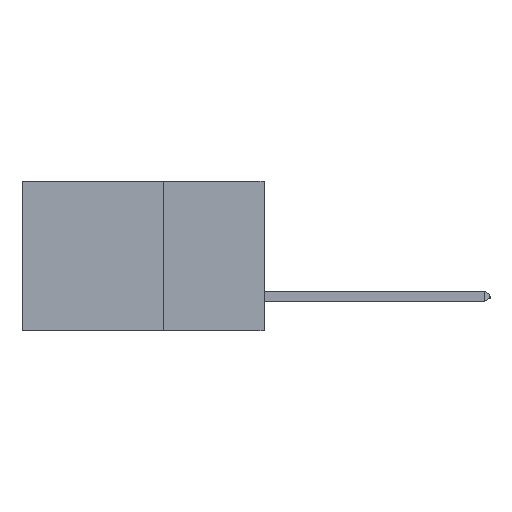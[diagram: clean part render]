
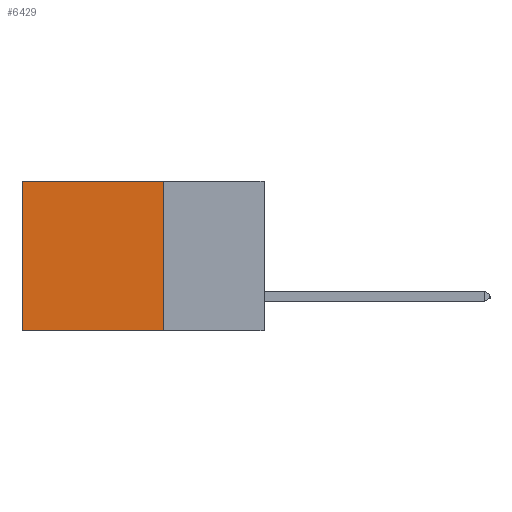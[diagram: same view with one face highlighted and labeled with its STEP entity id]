
A CAD part, left-side view. The second image highlights one B-rep face of the part: STEP entity #6429.
In plain terms, the highlighted planar face has unit normal (-1, 0, 0).
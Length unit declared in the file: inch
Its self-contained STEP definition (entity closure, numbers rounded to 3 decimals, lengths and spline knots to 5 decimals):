
#292 = AXIS2_PLACEMENT_3D ( 'NONE', #7613, #2351, #9661 ) ;
#304 = VECTOR ( 'NONE', #11605, 39.37008 ) ;
#675 = ORIENTED_EDGE ( 'NONE', *, *, #13280, .T. ) ;
#685 = DIRECTION ( 'NONE',  ( 0., 0., -1. ) ) ;
#794 = EDGE_CURVE ( 'NONE', #12680, #6023, #10056, .T. ) ;
#941 = CARTESIAN_POINT ( 'NONE',  ( 0.298, 0.25, 0. ) ) ;
#1238 = PLANE ( 'NONE',  #292 ) ;
#1508 = CARTESIAN_POINT ( 'NONE',  ( 0.298, 0.6, -0.37 ) ) ;
#2351 = DIRECTION ( 'NONE',  ( 1., 0., 0. ) ) ;
#2764 = CARTESIAN_POINT ( 'NONE',  ( 0.298, 0.25, -0.37 ) ) ;
#3000 = EDGE_LOOP ( 'NONE', ( #675, #11033, #6759, #5503 ) ) ;
#3111 = VERTEX_POINT ( 'NONE', #1508 ) ;
#3615 = CARTESIAN_POINT ( 'NONE',  ( 0.298, 0.25, 0. ) ) ;
#3887 = VECTOR ( 'NONE', #685, 39.37008 ) ;
#4018 = CARTESIAN_POINT ( 'NONE',  ( 0.298, 0.6, 0. ) ) ;
#4281 = VECTOR ( 'NONE', #13371, 39.37008 ) ;
#5053 = EDGE_CURVE ( 'NONE', #11545, #3111, #11174, .T. ) ;
#5503 = ORIENTED_EDGE ( 'NONE', *, *, #794, .T. ) ;
#6023 = VERTEX_POINT ( 'NONE', #9779 ) ;
#6429 = ADVANCED_FACE ( 'NONE', ( #7475 ), #1238, .F. ) ;
#6759 = ORIENTED_EDGE ( 'NONE', *, *, #10130, .F. ) ;
#7185 = CARTESIAN_POINT ( 'NONE',  ( 0.298, 0.25, 0. ) ) ;
#7475 = FACE_OUTER_BOUND ( 'NONE', #3000, .T. ) ;
#7613 = CARTESIAN_POINT ( 'NONE',  ( 0.298, 0.25, 0. ) ) ;
#7728 = DIRECTION ( 'NONE',  ( 0., 0., -1. ) ) ;
#9661 = DIRECTION ( 'NONE',  ( 0., 0., -1. ) ) ;
#9779 = CARTESIAN_POINT ( 'NONE',  ( 0.298, 0.6, 0. ) ) ;
#10056 = LINE ( 'NONE', #941, #4281 ) ;
#10130 = EDGE_CURVE ( 'NONE', #12680, #11545, #13199, .T. ) ;
#11033 = ORIENTED_EDGE ( 'NONE', *, *, #5053, .F. ) ;
#11174 = LINE ( 'NONE', #11622, #304 ) ;
#11545 = VERTEX_POINT ( 'NONE', #2764 ) ;
#11605 = DIRECTION ( 'NONE',  ( 0., 1., 0. ) ) ;
#11622 = CARTESIAN_POINT ( 'NONE',  ( 0.298, 0.25, -0.37 ) ) ;
#12021 = LINE ( 'NONE', #4018, #3887 ) ;
#12680 = VERTEX_POINT ( 'NONE', #7185 ) ;
#12882 = VECTOR ( 'NONE', #7728, 39.37008 ) ;
#13199 = LINE ( 'NONE', #3615, #12882 ) ;
#13280 = EDGE_CURVE ( 'NONE', #6023, #3111, #12021, .T. ) ;
#13371 = DIRECTION ( 'NONE',  ( 0., 1., 0. ) ) ;
